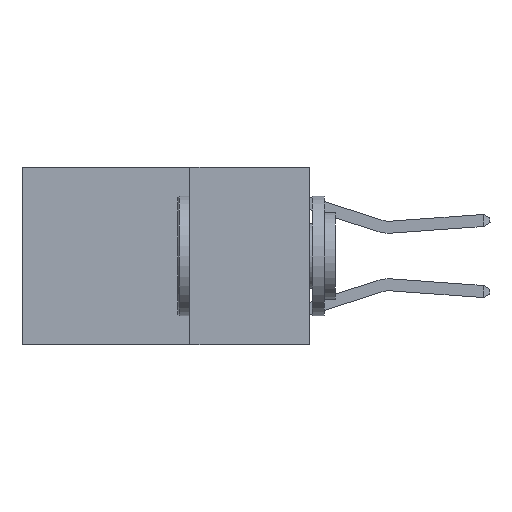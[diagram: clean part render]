
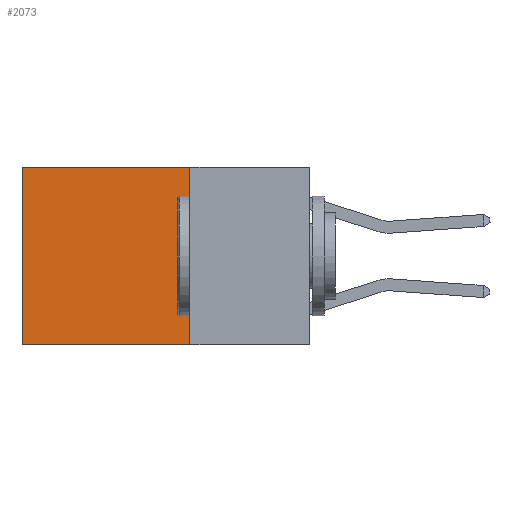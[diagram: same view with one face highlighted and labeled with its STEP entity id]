
A CAD part, left-side view. The second image highlights one B-rep face of the part: STEP entity #2073.
In plain terms, the highlighted planar face has unit normal (-1, 0, 0).
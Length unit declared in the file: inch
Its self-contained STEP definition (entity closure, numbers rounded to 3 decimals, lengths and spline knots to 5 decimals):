
#104 = DIRECTION ( 'NONE',  ( 1., 0., 0. ) ) ;
#804 = ORIENTED_EDGE ( 'NONE', *, *, #892, .F. ) ;
#892 = EDGE_CURVE ( 'NONE', #12240, #7626, #12964, .T. ) ;
#2073 = ADVANCED_FACE ( 'NONE', ( #5704 ), #6829, .F. ) ;
#2326 = EDGE_CURVE ( 'NONE', #7766, #7626, #3095, .T. ) ;
#2413 = ORIENTED_EDGE ( 'NONE', *, *, #3419, .F. ) ;
#2882 = AXIS2_PLACEMENT_3D ( 'NONE', #12253, #104, #7973 ) ;
#3095 = LINE ( 'NONE', #5556, #14177 ) ;
#3419 = EDGE_CURVE ( 'NONE', #12007, #12240, #13525, .T. ) ;
#3557 = LINE ( 'NONE', #13279, #9018 ) ;
#4477 = EDGE_CURVE ( 'NONE', #12007, #7766, #3557, .T. ) ;
#4628 = VECTOR ( 'NONE', #10875, 39.37008 ) ;
#4965 = ORIENTED_EDGE ( 'NONE', *, *, #2326, .T. ) ;
#5556 = CARTESIAN_POINT ( 'NONE',  ( 0.2625, 0.6, 0. ) ) ;
#5704 = FACE_OUTER_BOUND ( 'NONE', #9826, .T. ) ;
#5790 = DIRECTION ( 'NONE',  ( 0., 1., 0. ) ) ;
#6063 = CARTESIAN_POINT ( 'NONE',  ( 0.2625, 0.25, 0. ) ) ;
#6554 = CARTESIAN_POINT ( 'NONE',  ( 0.2625, 0.25, 0. ) ) ;
#6829 = PLANE ( 'NONE',  #2882 ) ;
#7626 = VERTEX_POINT ( 'NONE', #12307 ) ;
#7713 = DIRECTION ( 'NONE',  ( 0., 0., -1. ) ) ;
#7766 = VERTEX_POINT ( 'NONE', #8267 ) ;
#7973 = DIRECTION ( 'NONE',  ( 0., 0., -1. ) ) ;
#8021 = ORIENTED_EDGE ( 'NONE', *, *, #4477, .T. ) ;
#8267 = CARTESIAN_POINT ( 'NONE',  ( 0.2625, 0.6, 0. ) ) ;
#9018 = VECTOR ( 'NONE', #5790, 39.37008 ) ;
#9563 = DIRECTION ( 'NONE',  ( 0., 1., 0. ) ) ;
#9566 = CARTESIAN_POINT ( 'NONE',  ( 0.2625, 0.25, -0.37 ) ) ;
#9826 = EDGE_LOOP ( 'NONE', ( #4965, #804, #2413, #8021 ) ) ;
#10142 = VECTOR ( 'NONE', #9563, 39.37008 ) ;
#10324 = CARTESIAN_POINT ( 'NONE',  ( 0.2625, 0.25, -0.37 ) ) ;
#10875 = DIRECTION ( 'NONE',  ( 0., 0., -1. ) ) ;
#12007 = VERTEX_POINT ( 'NONE', #6063 ) ;
#12240 = VERTEX_POINT ( 'NONE', #9566 ) ;
#12253 = CARTESIAN_POINT ( 'NONE',  ( 0.2625, 0.25, 0. ) ) ;
#12307 = CARTESIAN_POINT ( 'NONE',  ( 0.2625, 0.6, -0.37 ) ) ;
#12964 = LINE ( 'NONE', #10324, #10142 ) ;
#13279 = CARTESIAN_POINT ( 'NONE',  ( 0.2625, 0.25, 0. ) ) ;
#13525 = LINE ( 'NONE', #6554, #4628 ) ;
#14177 = VECTOR ( 'NONE', #7713, 39.37008 ) ;
